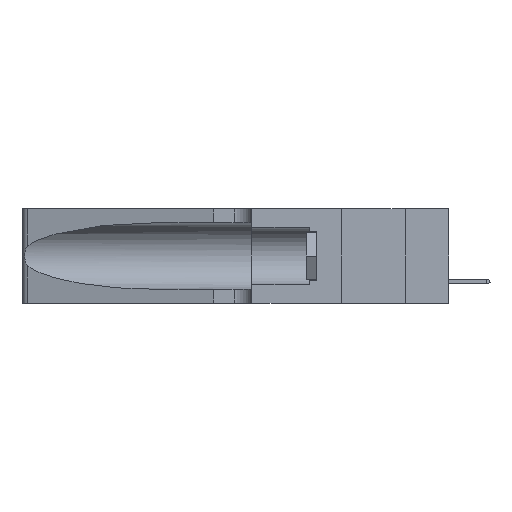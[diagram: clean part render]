
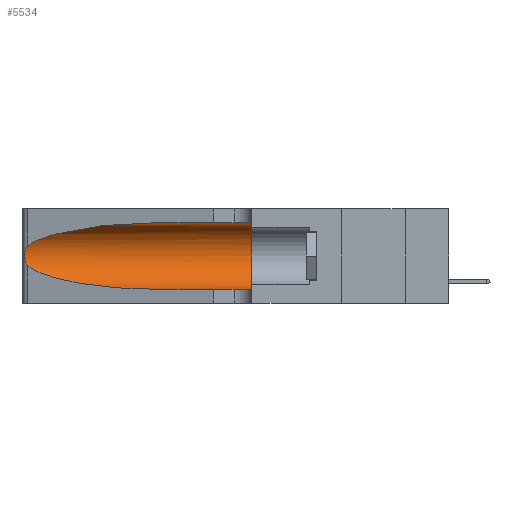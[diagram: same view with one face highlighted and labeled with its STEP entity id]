
A CAD part, left-side view. The second image highlights one B-rep face of the part: STEP entity #5534.
In plain terms, the highlighted cylindrical face has radius 3.308 mm (diameter 6.617 mm), a partial arc.
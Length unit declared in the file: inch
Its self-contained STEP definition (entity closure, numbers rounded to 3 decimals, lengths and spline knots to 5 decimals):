
#45 = CARTESIAN_POINT ( 'NONE',  ( 0.26017, 1.23833, 0.17102 ) ) ;
#50 = CARTESIAN_POINT ( 'NONE',  ( 0.1305, 1.61858, 0.05475 ) ) ;
#609 = ORIENTED_EDGE ( 'NONE', *, *, #3969, .T. ) ;
#660 = LINE ( 'NONE', #14223, #16248 ) ;
#707 = CARTESIAN_POINT ( 'NONE',  ( 0.1305, 0.72297, 0.31525 ) ) ;
#1020 = CARTESIAN_POINT ( 'NONE',  ( 0.18966, 0.96281, 0.31525 ) ) ;
#1232 = EDGE_CURVE ( 'NONE', #11894, #18203, #15453, .T. ) ;
#1494 = VERTEX_POINT ( 'NONE', #12944 ) ;
#1549 = EDGE_CURVE ( 'NONE', #21995, #18203, #11765, .T. ) ;
#1629 = FACE_OUTER_BOUND ( 'NONE', #20104, .T. ) ;
#1631 = CARTESIAN_POINT ( 'NONE',  ( 0.26018, 1.23835, 0.19895 ) ) ;
#2517 = CARTESIAN_POINT ( 'NONE',  ( 0.25487, 1.22718, 0.14631 ) ) ;
#3046 = EDGE_CURVE ( 'NONE', #5369, #1494, #20650, .T. ) ;
#3331 = DIRECTION ( 'NONE',  ( 0., 0., -1. ) ) ;
#3548 = CARTESIAN_POINT ( 'NONE',  ( 0.25787, 1.23484, 0.2124 ) ) ;
#3969 = EDGE_CURVE ( 'NONE', #1494, #11894, #21087, .T. ) ;
#4237 = CARTESIAN_POINT ( 'NONE',  ( 0.1305, 0.35, 0.31525 ) ) ;
#4659 = CARTESIAN_POINT ( 'NONE',  ( 0.25487, 1.22718, 0.22369 ) ) ;
#5289 = CARTESIAN_POINT ( 'NONE',  ( 0.26075, 1.23896, 0.19203 ) ) ;
#5363 = CARTESIAN_POINT ( 'NONE',  ( 0.25789, 1.23486, 0.15765 ) ) ;
#5369 = VERTEX_POINT ( 'NONE', #8949 ) ;
#5534 = ADVANCED_FACE ( 'NONE', ( #1629 ), #12131, .F. ) ;
#6203 = CARTESIAN_POINT ( 'NONE',  ( 0.1305, 0.35, 0.185 ) ) ;
#6688 = EDGE_CURVE ( 'NONE', #15420, #5369, #20800, .T. ) ;
#6895 = CARTESIAN_POINT ( 'NONE',  ( 0.1305, 0.72297, 0.05475 ) ) ;
#6928 = CARTESIAN_POINT ( 'NONE',  ( 0.1305, 0.72297, 0.05475 ) ) ;
#7190 = CARTESIAN_POINT ( 'NONE',  ( 0.25487, 1.22718, 0.14631 ) ) ;
#7365 = CARTESIAN_POINT ( 'NONE',  ( 0.25555, 1.22994, 0.2215 ) ) ;
#8222 = ORIENTED_EDGE ( 'NONE', *, *, #6688, .T. ) ;
#8827 = CARTESIAN_POINT ( 'NONE',  ( 0.18966, 0.96281, 0.05475 ) ) ;
#8949 = CARTESIAN_POINT ( 'NONE',  ( 0.25487, 1.22718, 0.22369 ) ) ;
#9156 = CARTESIAN_POINT ( 'NONE',  ( 0.25856, 1.23593, 0.16098 ) ) ;
#10662 = CARTESIAN_POINT ( 'NONE',  ( 0.25639, 1.23184, 0.21858 ) ) ;
#10802 = CARTESIAN_POINT ( 'NONE',  ( 0.1305, 0.35, 0.05475 ) ) ;
#10985 = CARTESIAN_POINT ( 'NONE',  ( 0.25555, 1.22993, 0.14849 ) ) ;
#11552 = DIRECTION ( 'NONE',  ( 0., -1., 0. ) ) ;
#11765 = CIRCLE ( 'NONE', #15220, 0.13025 ) ;
#11894 = VERTEX_POINT ( 'NONE', #6895 ) ;
#12069 = VECTOR ( 'NONE', #11552, 39.37008 ) ;
#12073 = CARTESIAN_POINT ( 'NONE',  ( 0.1305, 0.72297, 0.31525 ) ) ;
#12131 = CYLINDRICAL_SURFACE ( 'NONE', #17846, 0.13025 ) ;
#12393 = ORIENTED_EDGE ( 'NONE', *, *, #1232, .T. ) ;
#12944 = CARTESIAN_POINT ( 'NONE',  ( 0.25487, 1.22718, 0.14631 ) ) ;
#13621 = CARTESIAN_POINT ( 'NONE',  ( 0.2373, 1.15595, 0.28018 ) ) ;
#13820 = ORIENTED_EDGE ( 'NONE', *, *, #3046, .T. ) ;
#13868 = CARTESIAN_POINT ( 'NONE',  ( 0.1305, 1.61858, 0.185 ) ) ;
#14147 = DIRECTION ( 'NONE',  ( 0., -1., 0. ) ) ;
#14223 = CARTESIAN_POINT ( 'NONE',  ( 0.1305, 1.61858, 0.31525 ) ) ;
#14296 = CARTESIAN_POINT ( 'NONE',  ( 0.25639, 1.23186, 0.15144 ) ) ;
#14372 = CARTESIAN_POINT ( 'NONE',  ( 0.25487, 1.22718, 0.22369 ) ) ;
#15220 = AXIS2_PLACEMENT_3D ( 'NONE', #6203, #16833, #20699 ) ;
#15420 = VERTEX_POINT ( 'NONE', #12073 ) ;
#15453 = LINE ( 'NONE', #50, #12069 ) ;
#15950 = CARTESIAN_POINT ( 'NONE',  ( 0.2373, 1.15595, 0.08982 ) ) ;
#16248 = VECTOR ( 'NONE', #14147, 39.37008 ) ;
#16833 = DIRECTION ( 'NONE',  ( 0., 1., 0. ) ) ;
#17846 = AXIS2_PLACEMENT_3D ( 'NONE', #13868, #22959, #3331 ) ;
#17960 = CARTESIAN_POINT ( 'NONE',  ( 0.26075, 1.23896, 0.178 ) ) ;
#18203 = VERTEX_POINT ( 'NONE', #10802 ) ;
#20021 = CARTESIAN_POINT ( 'NONE',  ( 0.25854, 1.2359, 0.20912 ) ) ;
#20104 = EDGE_LOOP ( 'NONE', ( #8222, #13820, #609, #12393, #20593, #22779 ) ) ;
#20593 = ORIENTED_EDGE ( 'NONE', *, *, #1549, .F. ) ;
#20650 = B_SPLINE_CURVE_WITH_KNOTS ( 'NONE', 3,
 ( #14372, #7365, #10662, #3548, #20021, #1631, #5289, #17960, #45, #9156, #5363, #14296, #10985, #7190 ),
 .UNSPECIFIED., .F., .F.,
 ( 4, 2, 2, 2, 2, 2, 4 ),
 ( 0., 0.00027, 0.00053, 0.00107, 0.0016, 0.00187, 0.00214 ),
 .UNSPECIFIED. ) ;
#20699 = DIRECTION ( 'NONE',  ( 0., 0., 1. ) ) ;
#20800 =( BOUNDED_CURVE ( )  B_SPLINE_CURVE ( 3, ( #707, #1020, #13621, #4659 ),
 .UNSPECIFIED., .F., .F. ) 
 B_SPLINE_CURVE_WITH_KNOTS ( ( 4, 4 ),
 ( 1.5708, 2.84003 ),
 .UNSPECIFIED. ) 
 CURVE ( )  GEOMETRIC_REPRESENTATION_ITEM ( )  RATIONAL_B_SPLINE_CURVE ( ( 1., 0.87, 0.87, 1. ) ) 
 REPRESENTATION_ITEM ( '' )  );
#21043 = EDGE_CURVE ( 'NONE', #15420, #21995, #660, .T. ) ;
#21087 =( BOUNDED_CURVE ( )  B_SPLINE_CURVE ( 3, ( #2517, #15950, #8827, #6928 ),
 .UNSPECIFIED., .F., .T. ) 
 B_SPLINE_CURVE_WITH_KNOTS ( ( 4, 4 ),
 ( 3.44316, 4.71239 ),
 .UNSPECIFIED. ) 
 CURVE ( )  GEOMETRIC_REPRESENTATION_ITEM ( )  RATIONAL_B_SPLINE_CURVE ( ( 1., 0.87, 0.87, 1. ) ) 
 REPRESENTATION_ITEM ( '' )  );
#21995 = VERTEX_POINT ( 'NONE', #4237 ) ;
#22779 = ORIENTED_EDGE ( 'NONE', *, *, #21043, .F. ) ;
#22959 = DIRECTION ( 'NONE',  ( 0., -1., 0. ) ) ;
